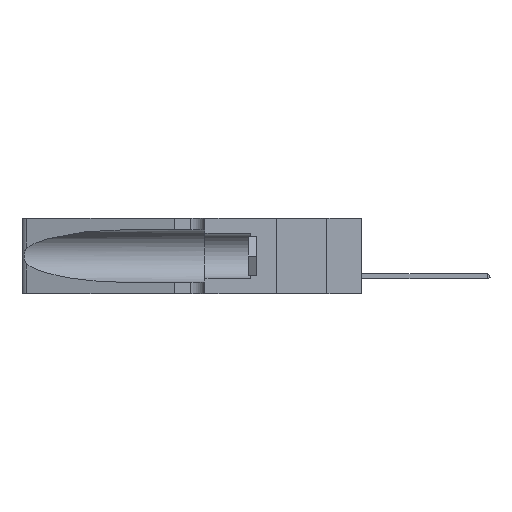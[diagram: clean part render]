
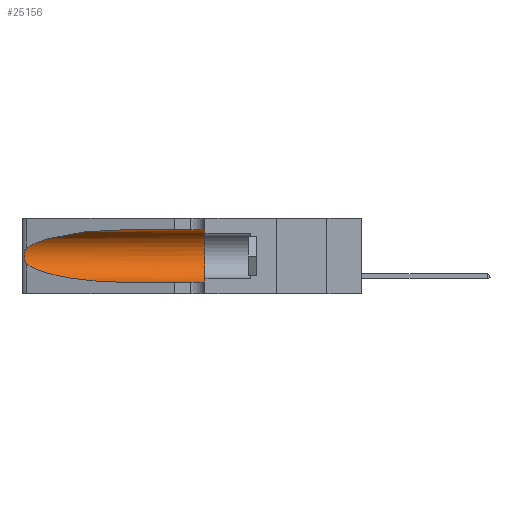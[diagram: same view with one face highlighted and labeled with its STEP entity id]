
A CAD part, left-side view. The second image highlights one B-rep face of the part: STEP entity #25156.
In plain terms, the highlighted cylindrical face has radius 3.308 mm (diameter 6.617 mm), a partial arc.
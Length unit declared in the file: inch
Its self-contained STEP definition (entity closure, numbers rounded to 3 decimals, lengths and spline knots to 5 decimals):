
#286 = EDGE_CURVE ( 'NONE', #5110, #26123, #19269, .T. ) ;
#806 = CARTESIAN_POINT ( 'NONE',  ( 0.26075, 1.23896, 0.178 ) ) ;
#1110 = CARTESIAN_POINT ( 'NONE',  ( 0.25639, 1.23184, 0.21858 ) ) ;
#1164 = VERTEX_POINT ( 'NONE', #26712 ) ;
#1807 = DIRECTION ( 'NONE',  ( 0., 0., -1. ) ) ;
#2120 = VECTOR ( 'NONE', #12280, 39.37008 ) ;
#2293 = CARTESIAN_POINT ( 'NONE',  ( 0.1305, 0.35, 0.31525 ) ) ;
#2799 = ORIENTED_EDGE ( 'NONE', *, *, #19191, .T. ) ;
#3312 = CARTESIAN_POINT ( 'NONE',  ( 0.25555, 1.22993, 0.14849 ) ) ;
#3520 = CARTESIAN_POINT ( 'NONE',  ( 0.25789, 1.23486, 0.15765 ) ) ;
#3690 =( BOUNDED_CURVE ( )  B_SPLINE_CURVE ( 3, ( #16489, #6604, #23277, #23481 ),
 .UNSPECIFIED., .F., .F. ) 
 B_SPLINE_CURVE_WITH_KNOTS ( ( 4, 4 ),
 ( 3.44316, 4.71239 ),
 .UNSPECIFIED. ) 
 CURVE ( )  GEOMETRIC_REPRESENTATION_ITEM ( )  RATIONAL_B_SPLINE_CURVE ( ( 1., 0.87, 0.87, 1. ) ) 
 REPRESENTATION_ITEM ( '' )  );
#3996 = VERTEX_POINT ( 'NONE', #13861 ) ;
#5110 = VERTEX_POINT ( 'NONE', #2293 ) ;
#5462 = LINE ( 'NONE', #14786, #2120 ) ;
#6014 = CARTESIAN_POINT ( 'NONE',  ( 0.25487, 1.22718, 0.22369 ) ) ;
#6049 = ORIENTED_EDGE ( 'NONE', *, *, #286, .F. ) ;
#6604 = CARTESIAN_POINT ( 'NONE',  ( 0.2373, 1.15595, 0.08982 ) ) ;
#8180 = CARTESIAN_POINT ( 'NONE',  ( 0.25856, 1.23593, 0.16098 ) ) ;
#10299 = CARTESIAN_POINT ( 'NONE',  ( 0.1305, 1.61858, 0.185 ) ) ;
#10453 = CARTESIAN_POINT ( 'NONE',  ( 0.25555, 1.22994, 0.2215 ) ) ;
#10668 = CARTESIAN_POINT ( 'NONE',  ( 0.25639, 1.23186, 0.15144 ) ) ;
#11134 = DIRECTION ( 'NONE',  ( 0., 1., 0. ) ) ;
#11425 = EDGE_CURVE ( 'NONE', #24114, #5110, #11427, .T. ) ;
#11427 = LINE ( 'NONE', #17270, #11789 ) ;
#11428 = EDGE_CURVE ( 'NONE', #1164, #26123, #5462, .T. ) ;
#11789 = VECTOR ( 'NONE', #17073, 39.37008 ) ;
#11918 = VERTEX_POINT ( 'NONE', #18699 ) ;
#12280 = DIRECTION ( 'NONE',  ( 0., -1., 0. ) ) ;
#12610 = CYLINDRICAL_SURFACE ( 'NONE', #24582, 0.13025 ) ;
#13861 = CARTESIAN_POINT ( 'NONE',  ( 0.25487, 1.22718, 0.14631 ) ) ;
#14307 = ORIENTED_EDGE ( 'NONE', *, *, #20625, .T. ) ;
#14786 = CARTESIAN_POINT ( 'NONE',  ( 0.1305, 1.61858, 0.05475 ) ) ;
#15135 = B_SPLINE_CURVE_WITH_KNOTS ( 'NONE', 3,
 ( #6014, #10453, #1110, #29607, #29504, #17663, #26936, #806, #17448, #8180, #3520, #10668, #3312, #27335 ),
 .UNSPECIFIED., .F., .F.,
 ( 4, 2, 2, 2, 2, 2, 4 ),
 ( 0., 0.00027, 0.00053, 0.00107, 0.0016, 0.00187, 0.00214 ),
 .UNSPECIFIED. ) ;
#15419 = CARTESIAN_POINT ( 'NONE',  ( 0.1305, 0.72297, 0.31525 ) ) ;
#16028 = AXIS2_PLACEMENT_3D ( 'NONE', #19382, #11134, #23232 ) ;
#16489 = CARTESIAN_POINT ( 'NONE',  ( 0.25487, 1.22718, 0.14631 ) ) ;
#17068 = ORIENTED_EDGE ( 'NONE', *, *, #11428, .T. ) ;
#17073 = DIRECTION ( 'NONE',  ( 0., -1., 0. ) ) ;
#17246 = EDGE_CURVE ( 'NONE', #11918, #3996, #15135, .T. ) ;
#17270 = CARTESIAN_POINT ( 'NONE',  ( 0.1305, 1.61858, 0.31525 ) ) ;
#17448 = CARTESIAN_POINT ( 'NONE',  ( 0.26017, 1.23833, 0.17102 ) ) ;
#17495 = CARTESIAN_POINT ( 'NONE',  ( 0.25487, 1.22718, 0.22369 ) ) ;
#17663 = CARTESIAN_POINT ( 'NONE',  ( 0.26018, 1.23835, 0.19895 ) ) ;
#18370 =( BOUNDED_CURVE ( )  B_SPLINE_CURVE ( 3, ( #15419, #20169, #29340, #17495 ),
 .UNSPECIFIED., .F., .F. ) 
 B_SPLINE_CURVE_WITH_KNOTS ( ( 4, 4 ),
 ( 1.5708, 2.84003 ),
 .UNSPECIFIED. ) 
 CURVE ( )  GEOMETRIC_REPRESENTATION_ITEM ( )  RATIONAL_B_SPLINE_CURVE ( ( 1., 0.87, 0.87, 1. ) ) 
 REPRESENTATION_ITEM ( '' )  );
#18699 = CARTESIAN_POINT ( 'NONE',  ( 0.25487, 1.22718, 0.22369 ) ) ;
#19191 = EDGE_CURVE ( 'NONE', #24114, #11918, #18370, .T. ) ;
#19269 = CIRCLE ( 'NONE', #16028, 0.13025 ) ;
#19382 = CARTESIAN_POINT ( 'NONE',  ( 0.1305, 0.35, 0.185 ) ) ;
#20169 = CARTESIAN_POINT ( 'NONE',  ( 0.18966, 0.96281, 0.31525 ) ) ;
#20625 = EDGE_CURVE ( 'NONE', #3996, #1164, #3690, .T. ) ;
#20824 = DIRECTION ( 'NONE',  ( 0., -1., 0. ) ) ;
#20995 = CARTESIAN_POINT ( 'NONE',  ( 0.1305, 0.72297, 0.31525 ) ) ;
#21534 = ORIENTED_EDGE ( 'NONE', *, *, #17246, .T. ) ;
#23232 = DIRECTION ( 'NONE',  ( 0., 0., 1. ) ) ;
#23277 = CARTESIAN_POINT ( 'NONE',  ( 0.18966, 0.96281, 0.05475 ) ) ;
#23481 = CARTESIAN_POINT ( 'NONE',  ( 0.1305, 0.72297, 0.05475 ) ) ;
#24114 = VERTEX_POINT ( 'NONE', #20995 ) ;
#24582 = AXIS2_PLACEMENT_3D ( 'NONE', #10299, #20824, #1807 ) ;
#25156 = ADVANCED_FACE ( 'NONE', ( #26358 ), #12610, .F. ) ;
#25491 = ORIENTED_EDGE ( 'NONE', *, *, #11425, .F. ) ;
#26123 = VERTEX_POINT ( 'NONE', #26491 ) ;
#26358 = FACE_OUTER_BOUND ( 'NONE', #30648, .T. ) ;
#26491 = CARTESIAN_POINT ( 'NONE',  ( 0.1305, 0.35, 0.05475 ) ) ;
#26712 = CARTESIAN_POINT ( 'NONE',  ( 0.1305, 0.72297, 0.05475 ) ) ;
#26936 = CARTESIAN_POINT ( 'NONE',  ( 0.26075, 1.23896, 0.19203 ) ) ;
#27335 = CARTESIAN_POINT ( 'NONE',  ( 0.25487, 1.22718, 0.14631 ) ) ;
#29340 = CARTESIAN_POINT ( 'NONE',  ( 0.2373, 1.15595, 0.28018 ) ) ;
#29504 = CARTESIAN_POINT ( 'NONE',  ( 0.25854, 1.2359, 0.20912 ) ) ;
#29607 = CARTESIAN_POINT ( 'NONE',  ( 0.25787, 1.23484, 0.2124 ) ) ;
#30648 = EDGE_LOOP ( 'NONE', ( #2799, #21534, #14307, #17068, #6049, #25491 ) ) ;
